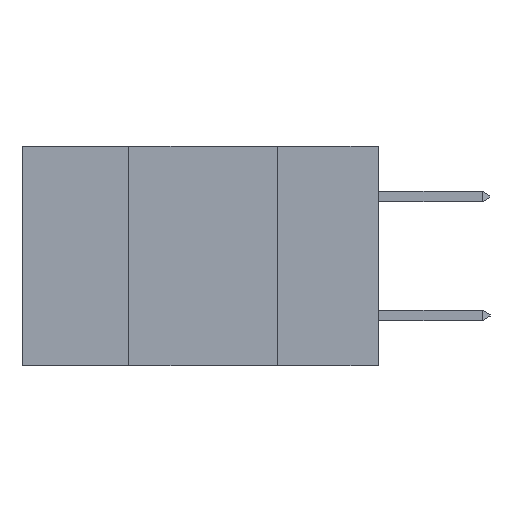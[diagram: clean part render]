
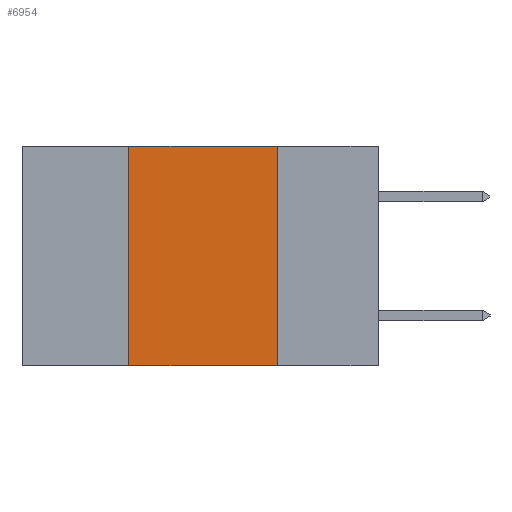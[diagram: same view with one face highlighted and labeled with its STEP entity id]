
A CAD part, left-side view. The second image highlights one B-rep face of the part: STEP entity #6954.
In plain terms, the highlighted planar face has unit normal (-1, 0, 0).
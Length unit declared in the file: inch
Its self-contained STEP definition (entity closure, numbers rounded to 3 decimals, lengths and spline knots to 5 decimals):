
#619 = ORIENTED_EDGE ( 'NONE', *, *, #14806, .T. ) ;
#738 = ORIENTED_EDGE ( 'NONE', *, *, #12485, .F. ) ;
#855 = ORIENTED_EDGE ( 'NONE', *, *, #10894, .F. ) ;
#912 = ORIENTED_EDGE ( 'NONE', *, *, #8443, .F. ) ;
#914 = CARTESIAN_POINT ( 'NONE',  ( 0., 0.42, -0.37 ) ) ;
#1453 = CARTESIAN_POINT ( 'NONE',  ( 0., 0.42, -0.37 ) ) ;
#1833 = CARTESIAN_POINT ( 'NONE',  ( 0., 0.42, 0. ) ) ;
#2195 = DIRECTION ( 'NONE',  ( 0., 0., 1. ) ) ;
#2704 = CARTESIAN_POINT ( 'NONE',  ( 0., 0.6, -0.37 ) ) ;
#2714 = VECTOR ( 'NONE', #3982, 39.37008 ) ;
#3429 = VECTOR ( 'NONE', #2195, 39.37008 ) ;
#3982 = DIRECTION ( 'NONE',  ( 0., -1., 0. ) ) ;
#5107 = CARTESIAN_POINT ( 'NONE',  ( 0., 0.17, -0.37 ) ) ;
#6438 = VERTEX_POINT ( 'NONE', #1453 ) ;
#6498 = CARTESIAN_POINT ( 'NONE',  ( 0., 0.17, 0. ) ) ;
#6954 = ADVANCED_FACE ( 'NONE', ( #14123 ), #10060, .F. ) ;
#7436 = EDGE_LOOP ( 'NONE', ( #912, #855, #738, #619 ) ) ;
#8443 = EDGE_CURVE ( 'NONE', #9761, #9808, #15149, .T. ) ;
#9307 = VERTEX_POINT ( 'NONE', #1833 ) ;
#9705 = DIRECTION ( 'NONE',  ( 0., 0., -1. ) ) ;
#9761 = VERTEX_POINT ( 'NONE', #6498 ) ;
#9783 = DIRECTION ( 'NONE',  ( 1., 0., 0. ) ) ;
#9808 = VERTEX_POINT ( 'NONE', #11351 ) ;
#9891 = AXIS2_PLACEMENT_3D ( 'NONE', #10099, #9783, #9705 ) ;
#10060 = PLANE ( 'NONE',  #9891 ) ;
#10099 = CARTESIAN_POINT ( 'NONE',  ( 0., 0.6, 0. ) ) ;
#10894 = EDGE_CURVE ( 'NONE', #9307, #9761, #11631, .T. ) ;
#11351 = CARTESIAN_POINT ( 'NONE',  ( 0., 0.17, -0.37 ) ) ;
#11631 = LINE ( 'NONE', #13885, #14358 ) ;
#12411 = LINE ( 'NONE', #2704, #2714 ) ;
#12485 = EDGE_CURVE ( 'NONE', #6438, #9307, #13052, .T. ) ;
#13052 = LINE ( 'NONE', #914, #3429 ) ;
#13531 = DIRECTION ( 'NONE',  ( 0., 0., -1. ) ) ;
#13885 = CARTESIAN_POINT ( 'NONE',  ( 0., 0.6, 0. ) ) ;
#14123 = FACE_OUTER_BOUND ( 'NONE', #7436, .T. ) ;
#14358 = VECTOR ( 'NONE', #15026, 39.37008 ) ;
#14804 = VECTOR ( 'NONE', #13531, 39.37008 ) ;
#14806 = EDGE_CURVE ( 'NONE', #6438, #9808, #12411, .T. ) ;
#15026 = DIRECTION ( 'NONE',  ( 0., -1., 0. ) ) ;
#15149 = LINE ( 'NONE', #5107, #14804 ) ;
